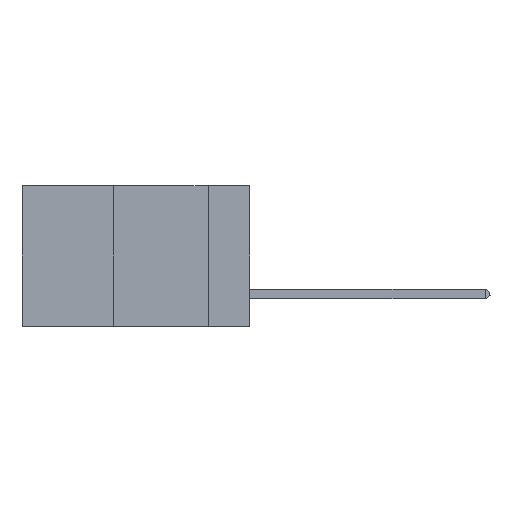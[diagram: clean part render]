
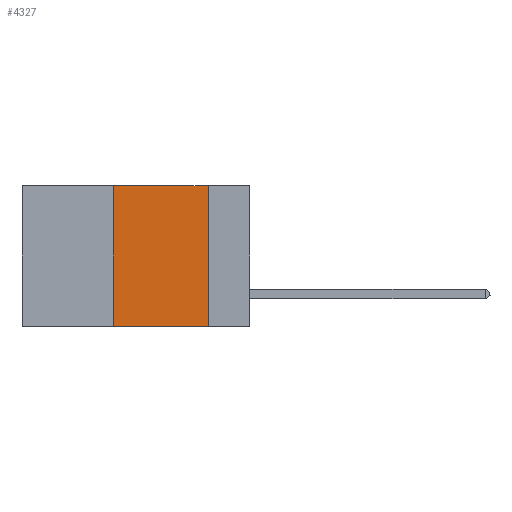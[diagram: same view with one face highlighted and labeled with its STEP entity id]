
A CAD part, left-side view. The second image highlights one B-rep face of the part: STEP entity #4327.
In plain terms, the highlighted planar face has unit normal (-1, 0, 0).
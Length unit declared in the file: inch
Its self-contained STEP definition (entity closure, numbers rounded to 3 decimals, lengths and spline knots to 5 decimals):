
#27 = EDGE_CURVE ( 'NONE', #5781, #7301, #8767, .T. ) ;
#1034 = CARTESIAN_POINT ( 'NONE',  ( 0., 0.36, 0. ) ) ;
#1526 = CARTESIAN_POINT ( 'NONE',  ( 0., 0.11, 0. ) ) ;
#1539 = VERTEX_POINT ( 'NONE', #3560 ) ;
#1546 = ORIENTED_EDGE ( 'NONE', *, *, #8718, .F. ) ;
#1607 = LINE ( 'NONE', #7230, #2227 ) ;
#1725 = AXIS2_PLACEMENT_3D ( 'NONE', #7504, #6174, #7470 ) ;
#1749 = CARTESIAN_POINT ( 'NONE',  ( 0., 0.36, 0. ) ) ;
#2227 = VECTOR ( 'NONE', #3188, 39.37008 ) ;
#2894 = DIRECTION ( 'NONE',  ( 0., -1., 0. ) ) ;
#3134 = ORIENTED_EDGE ( 'NONE', *, *, #4834, .T. ) ;
#3188 = DIRECTION ( 'NONE',  ( 0., -1., 0. ) ) ;
#3189 = VECTOR ( 'NONE', #5880, 39.37008 ) ;
#3332 = PLANE ( 'NONE',  #1725 ) ;
#3560 = CARTESIAN_POINT ( 'NONE',  ( 0., 0.36, -0.37 ) ) ;
#4327 = ADVANCED_FACE ( 'NONE', ( #5732 ), #3332, .F. ) ;
#4533 = VECTOR ( 'NONE', #2894, 39.37008 ) ;
#4622 = ORIENTED_EDGE ( 'NONE', *, *, #27, .F. ) ;
#4671 = CARTESIAN_POINT ( 'NONE',  ( 0., 0.11, 0. ) ) ;
#4738 = EDGE_LOOP ( 'NONE', ( #4622, #5683, #1546, #3134 ) ) ;
#4834 = EDGE_CURVE ( 'NONE', #1539, #7301, #8217, .T. ) ;
#5049 = VECTOR ( 'NONE', #6957, 39.37008 ) ;
#5683 = ORIENTED_EDGE ( 'NONE', *, *, #8208, .F. ) ;
#5693 = VERTEX_POINT ( 'NONE', #1034 ) ;
#5732 = FACE_OUTER_BOUND ( 'NONE', #4738, .T. ) ;
#5781 = VERTEX_POINT ( 'NONE', #4671 ) ;
#5880 = DIRECTION ( 'NONE',  ( 0., 0., 1. ) ) ;
#6174 = DIRECTION ( 'NONE',  ( 1., 0., 0. ) ) ;
#6266 = CARTESIAN_POINT ( 'NONE',  ( 0., 0.11, -0.37 ) ) ;
#6957 = DIRECTION ( 'NONE',  ( 0., 0., -1. ) ) ;
#7022 = CARTESIAN_POINT ( 'NONE',  ( 0., 0.6, -0.37 ) ) ;
#7230 = CARTESIAN_POINT ( 'NONE',  ( 0., 0.6, 0. ) ) ;
#7301 = VERTEX_POINT ( 'NONE', #6266 ) ;
#7470 = DIRECTION ( 'NONE',  ( 0., 0., -1. ) ) ;
#7504 = CARTESIAN_POINT ( 'NONE',  ( 0., 0.6, 0. ) ) ;
#7709 = LINE ( 'NONE', #1749, #3189 ) ;
#8208 = EDGE_CURVE ( 'NONE', #5693, #5781, #1607, .T. ) ;
#8217 = LINE ( 'NONE', #7022, #4533 ) ;
#8718 = EDGE_CURVE ( 'NONE', #1539, #5693, #7709, .T. ) ;
#8767 = LINE ( 'NONE', #1526, #5049 ) ;
